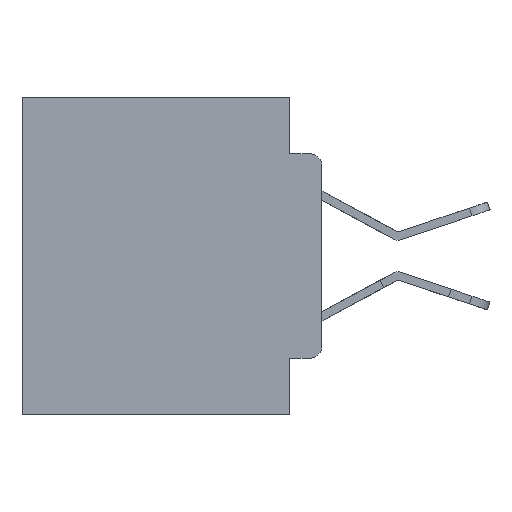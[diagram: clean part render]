
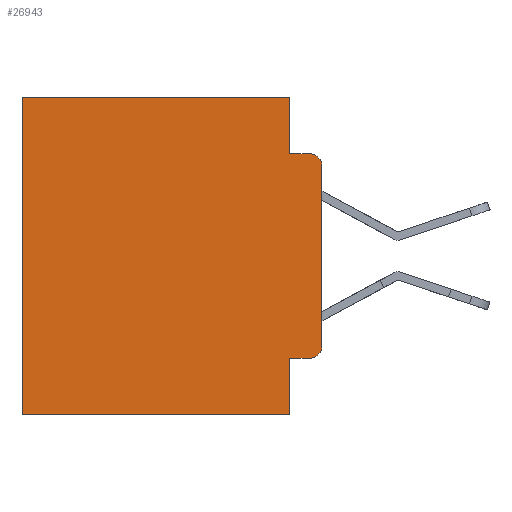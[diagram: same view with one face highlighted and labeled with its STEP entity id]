
A CAD part, left-side view. The second image highlights one B-rep face of the part: STEP entity #26943.
In plain terms, the highlighted planar face has unit normal (-1, 0, 0).
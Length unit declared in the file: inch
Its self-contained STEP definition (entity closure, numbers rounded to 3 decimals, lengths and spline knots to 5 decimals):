
#11 = VECTOR ( 'NONE', #20261, 39.37008 ) ;
#551 = DIRECTION ( 'NONE',  ( 0., -1., 0. ) ) ;
#640 = EDGE_CURVE ( 'NONE', #26263, #14340, #14796, .T. ) ;
#836 = CARTESIAN_POINT ( 'NONE',  ( 0.298, 0., -0.1085 ) ) ;
#943 = EDGE_CURVE ( 'NONE', #12787, #24990, #6340, .T. ) ;
#1069 = CARTESIAN_POINT ( 'NONE',  ( 0.298, 0.051, -0.4115 ) ) ;
#1555 = CARTESIAN_POINT ( 'NONE',  ( 0.298, 0.051, 0. ) ) ;
#1574 = CARTESIAN_POINT ( 'NONE',  ( 0.298, 0., 0. ) ) ;
#2500 = PLANE ( 'NONE',  #6782 ) ;
#3713 = CARTESIAN_POINT ( 'NONE',  ( 0.298, 0., -0.5 ) ) ;
#3773 = CARTESIAN_POINT ( 'NONE',  ( 0.298, 0.473, 0. ) ) ;
#3917 = DIRECTION ( 'NONE',  ( 0., 0., -1. ) ) ;
#3957 = VECTOR ( 'NONE', #3917, 39.37008 ) ;
#4179 = VECTOR ( 'NONE', #551, 39.37008 ) ;
#4881 = DIRECTION ( 'NONE',  ( -1., 0., 0. ) ) ;
#4998 = LINE ( 'NONE', #27012, #5708 ) ;
#5250 = DIRECTION ( 'NONE',  ( -1., 0., 0. ) ) ;
#5708 = VECTOR ( 'NONE', #7178, 39.37008 ) ;
#5994 = DIRECTION ( 'NONE',  ( 0., 1., 0. ) ) ;
#6114 = DIRECTION ( 'NONE',  ( 0., 0., -1. ) ) ;
#6340 = CIRCLE ( 'NONE', #22100, 0.02 ) ;
#6380 = VECTOR ( 'NONE', #8554, 39.37008 ) ;
#6782 = AXIS2_PLACEMENT_3D ( 'NONE', #22740, #9524, #24922 ) ;
#7173 = VERTEX_POINT ( 'NONE', #27646 ) ;
#7178 = DIRECTION ( 'NONE',  ( 0., 1., 0. ) ) ;
#7450 = FACE_OUTER_BOUND ( 'NONE', #10582, .T. ) ;
#7472 = ORIENTED_EDGE ( 'NONE', *, *, #9778, .F. ) ;
#7820 = ORIENTED_EDGE ( 'NONE', *, *, #10342, .T. ) ;
#8253 = VERTEX_POINT ( 'NONE', #25259 ) ;
#8554 = DIRECTION ( 'NONE',  ( 0., -1., 0. ) ) ;
#9033 = CARTESIAN_POINT ( 'NONE',  ( 0.298, 0.051, -0.0885 ) ) ;
#9102 = VERTEX_POINT ( 'NONE', #10621 ) ;
#9524 = DIRECTION ( 'NONE',  ( 1., 0., 0. ) ) ;
#9778 = EDGE_CURVE ( 'NONE', #9102, #7173, #14508, .T. ) ;
#9959 = ORIENTED_EDGE ( 'NONE', *, *, #943, .T. ) ;
#10010 = ORIENTED_EDGE ( 'NONE', *, *, #25372, .F. ) ;
#10342 = EDGE_CURVE ( 'NONE', #23766, #14340, #27107, .T. ) ;
#10582 = EDGE_LOOP ( 'NONE', ( #10010, #26615, #14536, #7472, #28373, #7820, #17329, #15599, #18593, #9959 ) ) ;
#10621 = CARTESIAN_POINT ( 'NONE',  ( 0.298, 0.051, 0. ) ) ;
#11968 = EDGE_CURVE ( 'NONE', #13431, #12787, #27056, .T. ) ;
#12178 = LINE ( 'NONE', #15856, #11 ) ;
#12787 = VERTEX_POINT ( 'NONE', #27825 ) ;
#12882 = DIRECTION ( 'NONE',  ( 0., 0., -1. ) ) ;
#13431 = VERTEX_POINT ( 'NONE', #1069 ) ;
#14340 = VERTEX_POINT ( 'NONE', #15291 ) ;
#14508 = LINE ( 'NONE', #1555, #20351 ) ;
#14536 = ORIENTED_EDGE ( 'NONE', *, *, #26801, .F. ) ;
#14796 = LINE ( 'NONE', #3713, #25735 ) ;
#15291 = CARTESIAN_POINT ( 'NONE',  ( 0.298, 0.473, -0.5 ) ) ;
#15515 = CIRCLE ( 'NONE', #21309, 0.02 ) ;
#15599 = ORIENTED_EDGE ( 'NONE', *, *, #18872, .F. ) ;
#15856 = CARTESIAN_POINT ( 'NONE',  ( 0.298, 0.051, 0. ) ) ;
#15940 = LINE ( 'NONE', #1574, #3957 ) ;
#15955 = CARTESIAN_POINT ( 'NONE',  ( 0.298, 0., -0.3915 ) ) ;
#17329 = ORIENTED_EDGE ( 'NONE', *, *, #640, .F. ) ;
#18410 = CARTESIAN_POINT ( 'NONE',  ( 0.298, 0.02, -0.3915 ) ) ;
#18593 = ORIENTED_EDGE ( 'NONE', *, *, #11968, .T. ) ;
#18667 = CARTESIAN_POINT ( 'NONE',  ( 0.298, 0.02, -0.1085 ) ) ;
#18872 = EDGE_CURVE ( 'NONE', #13431, #26263, #12178, .T. ) ;
#18945 = LINE ( 'NONE', #9033, #6380 ) ;
#20261 = DIRECTION ( 'NONE',  ( 0., 0., -1. ) ) ;
#20351 = VECTOR ( 'NONE', #6114, 39.37008 ) ;
#20515 = EDGE_CURVE ( 'NONE', #9102, #23766, #4998, .T. ) ;
#20728 = CARTESIAN_POINT ( 'NONE',  ( 0.298, 0.473, 0. ) ) ;
#20872 = DIRECTION ( 'NONE',  ( 0., 0., -1. ) ) ;
#20961 = DIRECTION ( 'NONE',  ( 0., 0., -1. ) ) ;
#21309 = AXIS2_PLACEMENT_3D ( 'NONE', #18667, #5250, #20872 ) ;
#21361 = VECTOR ( 'NONE', #12882, 39.37008 ) ;
#22100 = AXIS2_PLACEMENT_3D ( 'NONE', #18410, #4881, #20961 ) ;
#22740 = CARTESIAN_POINT ( 'NONE',  ( 0.298, 0., 0. ) ) ;
#23004 = CARTESIAN_POINT ( 'NONE',  ( 0.298, 0.051, -0.4115 ) ) ;
#23766 = VERTEX_POINT ( 'NONE', #20728 ) ;
#23896 = VERTEX_POINT ( 'NONE', #836 ) ;
#24922 = DIRECTION ( 'NONE',  ( 0., 0., -1. ) ) ;
#24990 = VERTEX_POINT ( 'NONE', #15955 ) ;
#25259 = CARTESIAN_POINT ( 'NONE',  ( 0.298, 0.02, -0.0885 ) ) ;
#25372 = EDGE_CURVE ( 'NONE', #23896, #24990, #15940, .T. ) ;
#25735 = VECTOR ( 'NONE', #5994, 39.37008 ) ;
#26263 = VERTEX_POINT ( 'NONE', #28650 ) ;
#26506 = EDGE_CURVE ( 'NONE', #23896, #8253, #15515, .T. ) ;
#26615 = ORIENTED_EDGE ( 'NONE', *, *, #26506, .T. ) ;
#26801 = EDGE_CURVE ( 'NONE', #7173, #8253, #18945, .T. ) ;
#26943 = ADVANCED_FACE ( 'NONE', ( #7450 ), #2500, .F. ) ;
#27012 = CARTESIAN_POINT ( 'NONE',  ( 0.298, 0., 0. ) ) ;
#27056 = LINE ( 'NONE', #23004, #4179 ) ;
#27107 = LINE ( 'NONE', #3773, #21361 ) ;
#27646 = CARTESIAN_POINT ( 'NONE',  ( 0.298, 0.051, -0.0885 ) ) ;
#27825 = CARTESIAN_POINT ( 'NONE',  ( 0.298, 0.02, -0.4115 ) ) ;
#28373 = ORIENTED_EDGE ( 'NONE', *, *, #20515, .T. ) ;
#28650 = CARTESIAN_POINT ( 'NONE',  ( 0.298, 0.051, -0.5 ) ) ;
